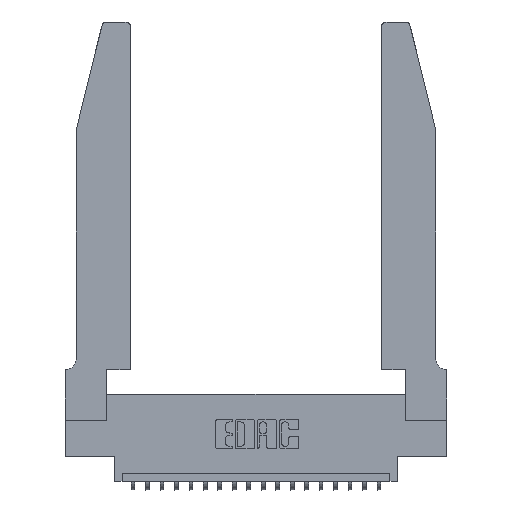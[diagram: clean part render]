
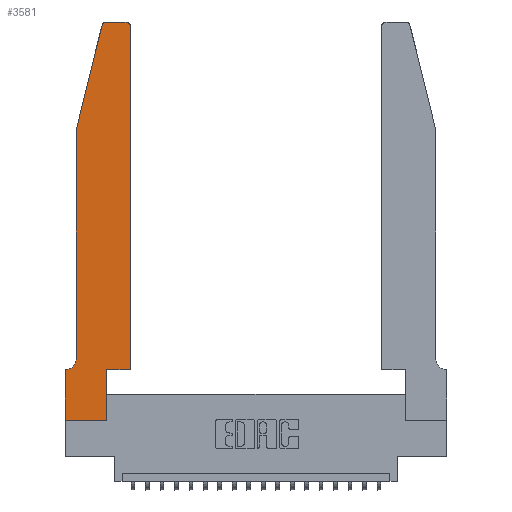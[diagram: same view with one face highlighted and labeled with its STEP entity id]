
A CAD part, top view. The second image highlights one B-rep face of the part: STEP entity #3581.
In plain terms, the highlighted planar face has unit normal (0, 0, 1).
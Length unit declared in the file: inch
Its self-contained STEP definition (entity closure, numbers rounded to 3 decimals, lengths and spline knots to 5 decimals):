
#580 = EDGE_CURVE ( 'NONE', #19027, #13609, #12182, .T. ) ;
#683 = DIRECTION ( 'NONE',  ( 0., 0., 1. ) ) ;
#941 = EDGE_CURVE ( 'NONE', #2121, #20155, #9798, .T. ) ;
#1106 = ORIENTED_EDGE ( 'NONE', *, *, #941, .T. ) ;
#2094 = AXIS2_PLACEMENT_3D ( 'NONE', #12033, #3326, #11892 ) ;
#2121 = VERTEX_POINT ( 'NONE', #14974 ) ;
#2195 = LINE ( 'NONE', #15587, #7129 ) ;
#2438 = CARTESIAN_POINT ( 'NONE',  ( 0.4505, 0.35, 0.37 ) ) ;
#2786 = DIRECTION ( 'NONE',  ( 0., 0., 1. ) ) ;
#2912 = CARTESIAN_POINT ( 'NONE',  ( 0.0755, 2., 0.37 ) ) ;
#2940 = CARTESIAN_POINT ( 'NONE',  ( 0.4205, 2.75, 0.37 ) ) ;
#3048 = VERTEX_POINT ( 'NONE', #11568 ) ;
#3054 = CARTESIAN_POINT ( 'NONE',  ( 0.4505, 0.35, 0.37 ) ) ;
#3148 = CARTESIAN_POINT ( 'NONE',  ( 0.2865, 0.35, 0.37 ) ) ;
#3288 = DIRECTION ( 'NONE',  ( -1., 0., 0. ) ) ;
#3326 = DIRECTION ( 'NONE',  ( 0., 0., 1. ) ) ;
#3373 = LINE ( 'NONE', #13403, #4926 ) ;
#3392 = DIRECTION ( 'NONE',  ( -0.239, -0.971, 0. ) ) ;
#3462 = EDGE_CURVE ( 'NONE', #20155, #18288, #10777, .T. ) ;
#3463 = CARTESIAN_POINT ( 'NONE',  ( 0.0755, 0.42, 0.37 ) ) ;
#3581 = ADVANCED_FACE ( 'NONE', ( #13616 ), #21402, .T. ) ;
#3877 = AXIS2_PLACEMENT_3D ( 'NONE', #13376, #13303, #3288 ) ;
#4926 = VECTOR ( 'NONE', #3392, 39.37008 ) ;
#5089 = ORIENTED_EDGE ( 'NONE', *, *, #18488, .T. ) ;
#5456 = LINE ( 'NONE', #2438, #14106 ) ;
#5653 = EDGE_CURVE ( 'NONE', #17773, #7712, #5456, .T. ) ;
#5851 = VECTOR ( 'NONE', #20498, 39.37008 ) ;
#5934 = EDGE_CURVE ( 'NONE', #13609, #3048, #3373, .T. ) ;
#7129 = VECTOR ( 'NONE', #18791, 39.37008 ) ;
#7712 = VERTEX_POINT ( 'NONE', #9700 ) ;
#8003 = DIRECTION ( 'NONE',  ( -1., 0., 0. ) ) ;
#8859 = CIRCLE ( 'NONE', #3877, 0.07 ) ;
#9638 = CARTESIAN_POINT ( 'NONE',  ( 0.2605, 2.75, 0.37 ) ) ;
#9700 = CARTESIAN_POINT ( 'NONE',  ( 0.4505, 0.35, 0.37 ) ) ;
#9783 = ORIENTED_EDGE ( 'NONE', *, *, #5934, .T. ) ;
#9798 = LINE ( 'NONE', #15933, #5851 ) ;
#10576 = ORIENTED_EDGE ( 'NONE', *, *, #17957, .T. ) ;
#10696 = CARTESIAN_POINT ( 'NONE',  ( 0.4205, 2.72, 0.37 ) ) ;
#10743 = ORIENTED_EDGE ( 'NONE', *, *, #20383, .T. ) ;
#10777 = LINE ( 'NONE', #14107, #16296 ) ;
#10902 = DIRECTION ( 'NONE',  ( 1., 0., 0. ) ) ;
#10999 = EDGE_CURVE ( 'NONE', #18288, #17773, #14600, .T. ) ;
#11182 = CARTESIAN_POINT ( 'NONE',  ( 0.2865, 0., 0.37 ) ) ;
#11321 = VERTEX_POINT ( 'NONE', #2940 ) ;
#11367 = DIRECTION ( 'NONE',  ( 0., 1., 0. ) ) ;
#11497 = ORIENTED_EDGE ( 'NONE', *, *, #20442, .T. ) ;
#11568 = CARTESIAN_POINT ( 'NONE',  ( 0.0755, 2., 0.37 ) ) ;
#11771 = VECTOR ( 'NONE', #8003, 39.37008 ) ;
#11892 = DIRECTION ( 'NONE',  ( 1., 0., 0. ) ) ;
#11901 = CARTESIAN_POINT ( 'NONE',  ( 0.4505, 2.72, 0.37 ) ) ;
#12033 = CARTESIAN_POINT ( 'NONE',  ( 0.284, 2.72, 0.37 ) ) ;
#12163 = CARTESIAN_POINT ( 'NONE',  ( 0., 0., 0.37 ) ) ;
#12170 = ORIENTED_EDGE ( 'NONE', *, *, #3462, .T. ) ;
#12182 = CIRCLE ( 'NONE', #2094, 0.03 ) ;
#12367 = DIRECTION ( 'NONE',  ( 1., 0., 0. ) ) ;
#12410 = VERTEX_POINT ( 'NONE', #19194 ) ;
#12905 = VERTEX_POINT ( 'NONE', #3463 ) ;
#13140 = DIRECTION ( 'NONE',  ( 0., 1., 0. ) ) ;
#13283 = CARTESIAN_POINT ( 'NONE',  ( 0.25487, 2.72718, 0.37 ) ) ;
#13303 = DIRECTION ( 'NONE',  ( 0., 0., -1. ) ) ;
#13376 = CARTESIAN_POINT ( 'NONE',  ( 0.0055, 0.42, 0.37 ) ) ;
#13403 = CARTESIAN_POINT ( 'NONE',  ( 0.0755, 2., 0.37 ) ) ;
#13439 = ORIENTED_EDGE ( 'NONE', *, *, #10999, .T. ) ;
#13609 = VERTEX_POINT ( 'NONE', #13283 ) ;
#13616 = FACE_OUTER_BOUND ( 'NONE', #19516, .T. ) ;
#13704 = ORIENTED_EDGE ( 'NONE', *, *, #14180, .T. ) ;
#13813 = EDGE_CURVE ( 'NONE', #3048, #12905, #17742, .T. ) ;
#14003 = ORIENTED_EDGE ( 'NONE', *, *, #580, .T. ) ;
#14106 = VECTOR ( 'NONE', #18946, 39.37008 ) ;
#14107 = CARTESIAN_POINT ( 'NONE',  ( 0., 0., 0.37 ) ) ;
#14135 = VERTEX_POINT ( 'NONE', #11901 ) ;
#14180 = EDGE_CURVE ( 'NONE', #7712, #14135, #16935, .T. ) ;
#14552 = CARTESIAN_POINT ( 'NONE',  ( 0., 0.35, 0.37 ) ) ;
#14600 = LINE ( 'NONE', #15019, #18028 ) ;
#14637 = LINE ( 'NONE', #9638, #11771 ) ;
#14974 = CARTESIAN_POINT ( 'NONE',  ( 0., 0.35, 0.37 ) ) ;
#15019 = CARTESIAN_POINT ( 'NONE',  ( 0.2865, 0.35, 0.37 ) ) ;
#15287 = CIRCLE ( 'NONE', #21423, 0.03 ) ;
#15587 = CARTESIAN_POINT ( 'NONE',  ( 0.0755, 0.35, 0.37 ) ) ;
#15933 = CARTESIAN_POINT ( 'NONE',  ( 0., 0., 0.37 ) ) ;
#16296 = VECTOR ( 'NONE', #10902, 39.37008 ) ;
#16389 = VECTOR ( 'NONE', #13140, 39.37008 ) ;
#16396 = DIRECTION ( 'NONE',  ( 1., 0., 0. ) ) ;
#16935 = LINE ( 'NONE', #3054, #16389 ) ;
#17227 = CARTESIAN_POINT ( 'NONE',  ( 0.284, 2.75, 0.37 ) ) ;
#17742 = LINE ( 'NONE', #2912, #20890 ) ;
#17773 = VERTEX_POINT ( 'NONE', #3148 ) ;
#17957 = EDGE_CURVE ( 'NONE', #12410, #2121, #2195, .T. ) ;
#18028 = VECTOR ( 'NONE', #11367, 39.37008 ) ;
#18288 = VERTEX_POINT ( 'NONE', #11182 ) ;
#18488 = EDGE_CURVE ( 'NONE', #14135, #11321, #15287, .T. ) ;
#18791 = DIRECTION ( 'NONE',  ( -1., 0., 0. ) ) ;
#18946 = DIRECTION ( 'NONE',  ( 1., 0., 0. ) ) ;
#19027 = VERTEX_POINT ( 'NONE', #17227 ) ;
#19194 = CARTESIAN_POINT ( 'NONE',  ( 0.0055, 0.35, 0.37 ) ) ;
#19516 = EDGE_LOOP ( 'NONE', ( #10743, #14003, #9783, #20026, #11497, #10576, #1106, #12170, #13439, #21770, #13704, #5089 ) ) ;
#20026 = ORIENTED_EDGE ( 'NONE', *, *, #13813, .T. ) ;
#20155 = VERTEX_POINT ( 'NONE', #12163 ) ;
#20212 = DIRECTION ( 'NONE',  ( 0., -1., 0. ) ) ;
#20383 = EDGE_CURVE ( 'NONE', #11321, #19027, #14637, .T. ) ;
#20442 = EDGE_CURVE ( 'NONE', #12905, #12410, #8859, .T. ) ;
#20498 = DIRECTION ( 'NONE',  ( 0., -1., 0. ) ) ;
#20530 = AXIS2_PLACEMENT_3D ( 'NONE', #14552, #2786, #16396 ) ;
#20890 = VECTOR ( 'NONE', #20212, 39.37008 ) ;
#21402 = PLANE ( 'NONE',  #20530 ) ;
#21423 = AXIS2_PLACEMENT_3D ( 'NONE', #10696, #683, #12367 ) ;
#21770 = ORIENTED_EDGE ( 'NONE', *, *, #5653, .T. ) ;
